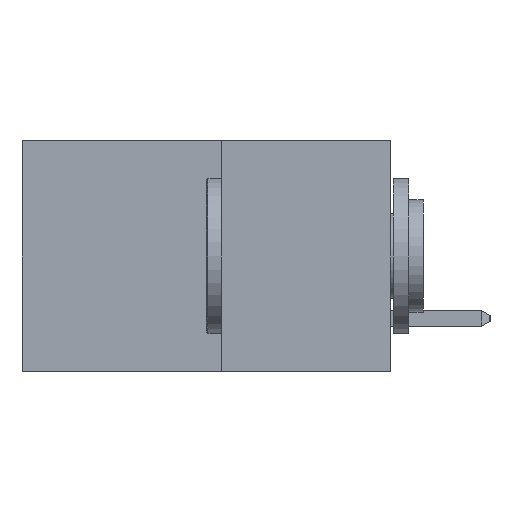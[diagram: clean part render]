
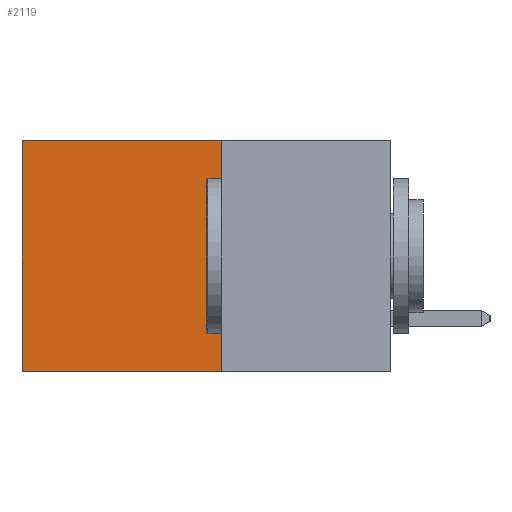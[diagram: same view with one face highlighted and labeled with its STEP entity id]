
A CAD part, left-side view. The second image highlights one B-rep face of the part: STEP entity #2119.
In plain terms, the highlighted planar face has unit normal (-1, 0, 0).
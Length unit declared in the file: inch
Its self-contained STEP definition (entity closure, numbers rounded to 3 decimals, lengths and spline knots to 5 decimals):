
#499 = LINE ( 'NONE', #12886, #6394 ) ;
#1101 = VECTOR ( 'NONE', #5303, 39.37008 ) ;
#1611 = AXIS2_PLACEMENT_3D ( 'NONE', #6001, #12106, #14554 ) ;
#1651 = ORIENTED_EDGE ( 'NONE', *, *, #4627, .T. ) ;
#1657 = VERTEX_POINT ( 'NONE', #6563 ) ;
#2119 = ADVANCED_FACE ( 'NONE', ( #12507 ), #10908, .F. ) ;
#2830 = CARTESIAN_POINT ( 'NONE',  ( 0.277, 0.27, -0.37 ) ) ;
#3143 = VERTEX_POINT ( 'NONE', #11764 ) ;
#3390 = ORIENTED_EDGE ( 'NONE', *, *, #9981, .T. ) ;
#4055 = DIRECTION ( 'NONE',  ( 0., 0., -1. ) ) ;
#4393 = EDGE_LOOP ( 'NONE', ( #3390, #13542, #4552, #1651 ) ) ;
#4552 = ORIENTED_EDGE ( 'NONE', *, *, #5835, .F. ) ;
#4627 = EDGE_CURVE ( 'NONE', #3143, #5658, #10061, .T. ) ;
#5103 = DIRECTION ( 'NONE',  ( 0., 1., 0. ) ) ;
#5284 = CARTESIAN_POINT ( 'NONE',  ( 0.277, 0.27, -0.37 ) ) ;
#5303 = DIRECTION ( 'NONE',  ( 0., 0., -1. ) ) ;
#5471 = CARTESIAN_POINT ( 'NONE',  ( 0.277, 0.27, 0. ) ) ;
#5658 = VERTEX_POINT ( 'NONE', #6849 ) ;
#5776 = DIRECTION ( 'NONE',  ( 0., 1., 0. ) ) ;
#5835 = EDGE_CURVE ( 'NONE', #3143, #7593, #13494, .T. ) ;
#6001 = CARTESIAN_POINT ( 'NONE',  ( 0.277, 0.27, -0.37 ) ) ;
#6394 = VECTOR ( 'NONE', #5103, 39.37008 ) ;
#6563 = CARTESIAN_POINT ( 'NONE',  ( 0.277, 0.59, -0.37 ) ) ;
#6729 = VECTOR ( 'NONE', #5776, 39.37008 ) ;
#6849 = CARTESIAN_POINT ( 'NONE',  ( 0.277, 0.59, 0. ) ) ;
#7593 = VERTEX_POINT ( 'NONE', #2830 ) ;
#8547 = CARTESIAN_POINT ( 'NONE',  ( 0.277, 0.59, -0.37 ) ) ;
#9981 = EDGE_CURVE ( 'NONE', #5658, #1657, #13222, .T. ) ;
#10061 = LINE ( 'NONE', #5471, #6729 ) ;
#10346 = VECTOR ( 'NONE', #4055, 39.37008 ) ;
#10908 = PLANE ( 'NONE',  #1611 ) ;
#11764 = CARTESIAN_POINT ( 'NONE',  ( 0.277, 0.27, 0. ) ) ;
#11894 = EDGE_CURVE ( 'NONE', #7593, #1657, #499, .T. ) ;
#12106 = DIRECTION ( 'NONE',  ( 1., 0., 0. ) ) ;
#12507 = FACE_OUTER_BOUND ( 'NONE', #4393, .T. ) ;
#12886 = CARTESIAN_POINT ( 'NONE',  ( 0.277, 0.27, -0.37 ) ) ;
#13222 = LINE ( 'NONE', #8547, #10346 ) ;
#13494 = LINE ( 'NONE', #5284, #1101 ) ;
#13542 = ORIENTED_EDGE ( 'NONE', *, *, #11894, .F. ) ;
#14554 = DIRECTION ( 'NONE',  ( 0., 0., -1. ) ) ;
